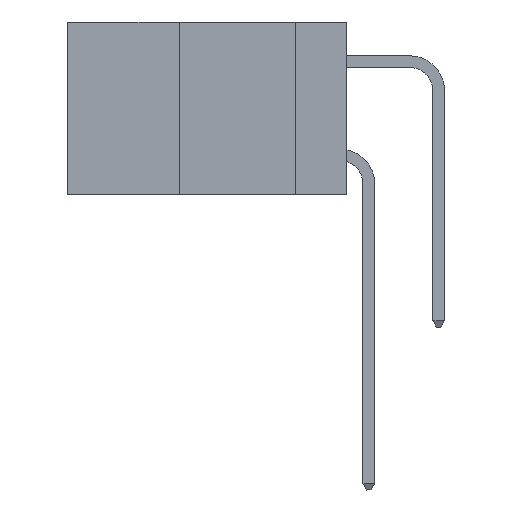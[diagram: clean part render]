
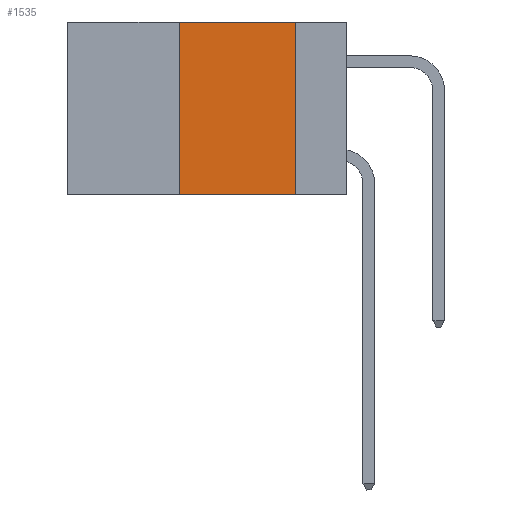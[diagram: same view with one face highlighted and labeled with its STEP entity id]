
A CAD part, left-side view. The second image highlights one B-rep face of the part: STEP entity #1535.
In plain terms, the highlighted planar face has unit normal (-1, 0, 0).
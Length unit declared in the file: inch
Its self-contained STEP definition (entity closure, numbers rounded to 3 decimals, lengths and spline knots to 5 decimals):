
#901 = EDGE_CURVE ( 'NONE', #1414, #23038, #16457, .T. ) ;
#1167 = VERTEX_POINT ( 'NONE', #8844 ) ;
#1359 = CARTESIAN_POINT ( 'NONE',  ( 0., 0.11, -0.37 ) ) ;
#1414 = VERTEX_POINT ( 'NONE', #17038 ) ;
#1535 = ADVANCED_FACE ( 'NONE', ( #6759 ), #9879, .F. ) ;
#1551 = VECTOR ( 'NONE', #15574, 39.37008 ) ;
#2361 = VECTOR ( 'NONE', #12090, 39.37008 ) ;
#2458 = CARTESIAN_POINT ( 'NONE',  ( 0., 0.6, 0. ) ) ;
#3055 = DIRECTION ( 'NONE',  ( 0., 0., 1. ) ) ;
#4338 = DIRECTION ( 'NONE',  ( 0., 0., -1. ) ) ;
#4467 = VECTOR ( 'NONE', #3055, 39.37008 ) ;
#6744 = LINE ( 'NONE', #17767, #2361 ) ;
#6759 = FACE_OUTER_BOUND ( 'NONE', #9666, .T. ) ;
#8279 = ORIENTED_EDGE ( 'NONE', *, *, #901, .F. ) ;
#8579 = ORIENTED_EDGE ( 'NONE', *, *, #13024, .F. ) ;
#8844 = CARTESIAN_POINT ( 'NONE',  ( 0., 0.36, -0.37 ) ) ;
#9666 = EDGE_LOOP ( 'NONE', ( #8279, #8579, #10352, #12657 ) ) ;
#9879 = PLANE ( 'NONE',  #20803 ) ;
#10352 = ORIENTED_EDGE ( 'NONE', *, *, #11679, .F. ) ;
#10590 = DIRECTION ( 'NONE',  ( 0., -1., 0. ) ) ;
#11679 = EDGE_CURVE ( 'NONE', #1167, #12489, #19390, .T. ) ;
#12090 = DIRECTION ( 'NONE',  ( 0., -1., 0. ) ) ;
#12395 = CARTESIAN_POINT ( 'NONE',  ( 0., 0.36, 0. ) ) ;
#12489 = VERTEX_POINT ( 'NONE', #23856 ) ;
#12657 = ORIENTED_EDGE ( 'NONE', *, *, #12893, .T. ) ;
#12893 = EDGE_CURVE ( 'NONE', #1167, #23038, #6744, .T. ) ;
#13024 = EDGE_CURVE ( 'NONE', #12489, #1414, #13795, .T. ) ;
#13795 = LINE ( 'NONE', #18080, #23043 ) ;
#15543 = DIRECTION ( 'NONE',  ( 1., 0., 0. ) ) ;
#15574 = DIRECTION ( 'NONE',  ( 0., 0., -1. ) ) ;
#16457 = LINE ( 'NONE', #19249, #1551 ) ;
#17038 = CARTESIAN_POINT ( 'NONE',  ( 0., 0.11, 0. ) ) ;
#17767 = CARTESIAN_POINT ( 'NONE',  ( 0., 0.6, -0.37 ) ) ;
#18080 = CARTESIAN_POINT ( 'NONE',  ( 0., 0.6, 0. ) ) ;
#19249 = CARTESIAN_POINT ( 'NONE',  ( 0., 0.11, 0. ) ) ;
#19390 = LINE ( 'NONE', #12395, #4467 ) ;
#20803 = AXIS2_PLACEMENT_3D ( 'NONE', #2458, #15543, #4338 ) ;
#23038 = VERTEX_POINT ( 'NONE', #1359 ) ;
#23043 = VECTOR ( 'NONE', #10590, 39.37008 ) ;
#23856 = CARTESIAN_POINT ( 'NONE',  ( 0., 0.36, 0. ) ) ;
